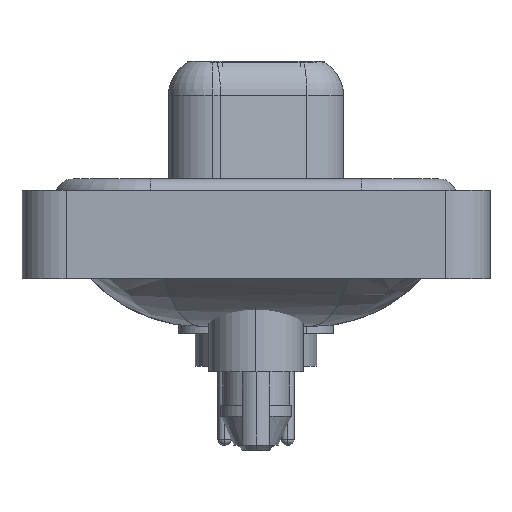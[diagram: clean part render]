
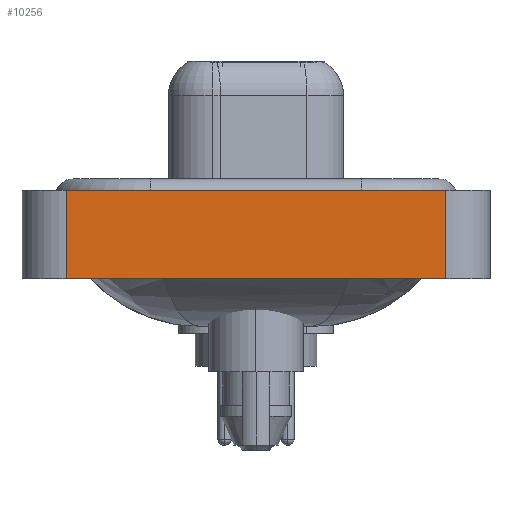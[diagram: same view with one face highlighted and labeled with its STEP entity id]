
A CAD part, left-side view. The second image highlights one B-rep face of the part: STEP entity #10256.
In plain terms, the highlighted planar face has unit normal (-1, 0, 0).
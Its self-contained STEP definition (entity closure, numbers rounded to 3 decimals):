
#66 = CARTESIAN_POINT ( 'NONE',  ( -7.35, -8.55, -3.6 ) ) ;
#872 = VERTEX_POINT ( 'NONE', #16921 ) ;
#1127 = CARTESIAN_POINT ( 'NONE',  ( -7.35, 8.55, -3.6 ) ) ;
#1261 = EDGE_CURVE ( 'NONE', #22550, #1291, #16998, .T. ) ;
#1291 = VERTEX_POINT ( 'NONE', #7881 ) ;
#1609 = LINE ( 'NONE', #14155, #3587 ) ;
#3527 = ORIENTED_EDGE ( 'NONE', *, *, #1261, .F. ) ;
#3587 = VECTOR ( 'NONE', #5148, 1000. ) ;
#4141 = EDGE_CURVE ( 'NONE', #872, #22550, #22835, .T. ) ;
#4257 = EDGE_CURVE ( 'NONE', #14973, #1291, #1609, .T. ) ;
#4355 = DIRECTION ( 'NONE',  ( -1., 0., 0. ) ) ;
#5148 = DIRECTION ( 'NONE',  ( 0., 0., 1. ) ) ;
#5260 = DIRECTION ( 'NONE',  ( 0., 0., 1. ) ) ;
#6120 = FACE_OUTER_BOUND ( 'NONE', #16190, .T. ) ;
#6322 = CARTESIAN_POINT ( 'NONE',  ( -7.35, 8.55, 0.4 ) ) ;
#7264 = VECTOR ( 'NONE', #20584, 1000. ) ;
#7881 = CARTESIAN_POINT ( 'NONE',  ( -7.35, -8.55, 0.4 ) ) ;
#10256 = ADVANCED_FACE ( 'NONE', ( #6120 ), #13242, .T. ) ;
#10823 = ORIENTED_EDGE ( 'NONE', *, *, #4257, .T. ) ;
#10942 = DIRECTION ( 'NONE',  ( 0., -1., 0. ) ) ;
#11270 = AXIS2_PLACEMENT_3D ( 'NONE', #17134, #4355, #22495 ) ;
#13242 = PLANE ( 'NONE',  #11270 ) ;
#13310 = ORIENTED_EDGE ( 'NONE', *, *, #4141, .F. ) ;
#13858 = CARTESIAN_POINT ( 'NONE',  ( -7.35, -8.55, -3.6 ) ) ;
#14155 = CARTESIAN_POINT ( 'NONE',  ( -7.35, -8.55, -3.6 ) ) ;
#14973 = VERTEX_POINT ( 'NONE', #13858 ) ;
#16040 = EDGE_CURVE ( 'NONE', #872, #14973, #16266, .T. ) ;
#16190 = EDGE_LOOP ( 'NONE', ( #10823, #3527, #13310, #19586 ) ) ;
#16266 = LINE ( 'NONE', #66, #22086 ) ;
#16921 = CARTESIAN_POINT ( 'NONE',  ( -7.35, 8.55, -3.6 ) ) ;
#16998 = LINE ( 'NONE', #20692, #7264 ) ;
#17134 = CARTESIAN_POINT ( 'NONE',  ( -7.35, -8.55, -3.6 ) ) ;
#19477 = VECTOR ( 'NONE', #5260, 1000. ) ;
#19586 = ORIENTED_EDGE ( 'NONE', *, *, #16040, .T. ) ;
#20584 = DIRECTION ( 'NONE',  ( 0., -1., 0. ) ) ;
#20692 = CARTESIAN_POINT ( 'NONE',  ( -7.35, -8.55, 0.4 ) ) ;
#22086 = VECTOR ( 'NONE', #10942, 1000. ) ;
#22495 = DIRECTION ( 'NONE',  ( 0., 0., 1. ) ) ;
#22550 = VERTEX_POINT ( 'NONE', #6322 ) ;
#22835 = LINE ( 'NONE', #1127, #19477 ) ;
